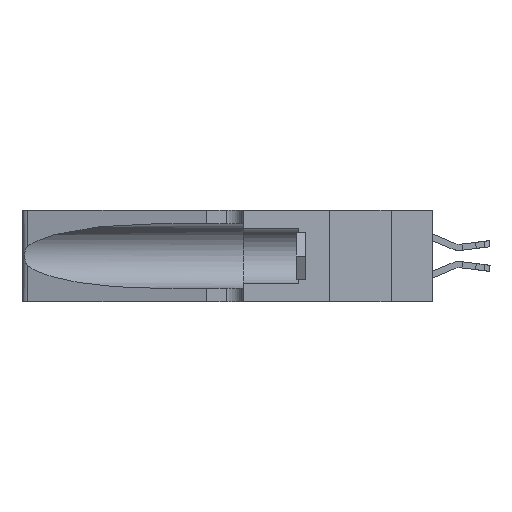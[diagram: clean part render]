
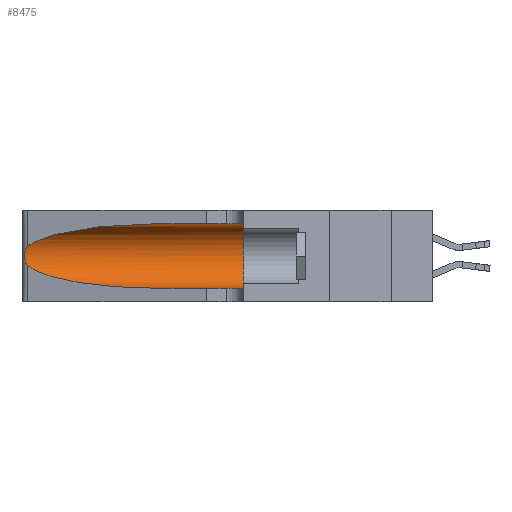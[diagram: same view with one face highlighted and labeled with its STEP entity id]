
A CAD part, left-side view. The second image highlights one B-rep face of the part: STEP entity #8475.
In plain terms, the highlighted cylindrical face has radius 3.308 mm (diameter 6.617 mm), a partial arc.
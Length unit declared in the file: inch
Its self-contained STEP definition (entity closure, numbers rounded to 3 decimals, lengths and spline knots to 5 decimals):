
#1839 = CARTESIAN_POINT ( 'NONE',  ( 0.1305, 0.35, 0.05475 ) ) ;
#1870 = CARTESIAN_POINT ( 'NONE',  ( 0.2373, 1.15595, 0.08982 ) ) ;
#2159 = CARTESIAN_POINT ( 'NONE',  ( 0.25856, 1.23593, 0.16098 ) ) ;
#3653 = LINE ( 'NONE', #21757, #31577 ) ;
#3708 = DIRECTION ( 'NONE',  ( 0., -1., 0. ) ) ;
#4135 = EDGE_CURVE ( 'NONE', #25041, #7422, #7489, .T. ) ;
#5105 = VECTOR ( 'NONE', #11735, 39.37008 ) ;
#5271 = CARTESIAN_POINT ( 'NONE',  ( 0.1305, 0.72297, 0.31525 ) ) ;
#5414 = VERTEX_POINT ( 'NONE', #26259 ) ;
#5548 = ORIENTED_EDGE ( 'NONE', *, *, #18888, .F. ) ;
#6478 = DIRECTION ( 'NONE',  ( 0., 1., 0. ) ) ;
#7023 = CARTESIAN_POINT ( 'NONE',  ( 0.25639, 1.23186, 0.15144 ) ) ;
#7106 = FACE_OUTER_BOUND ( 'NONE', #10210, .T. ) ;
#7422 = VERTEX_POINT ( 'NONE', #12897 ) ;
#7489 = B_SPLINE_CURVE_WITH_KNOTS ( 'NONE', 3,
 ( #26254, #9355, #31167, #16526, #26468, #31381, #23822, #11772, #9252, #2159, #31061, #7023, #16828, #28608 ),
 .UNSPECIFIED., .F., .F.,
 ( 4, 2, 2, 2, 2, 2, 4 ),
 ( 0., 0.00027, 0.00053, 0.00107, 0.0016, 0.00187, 0.00214 ),
 .UNSPECIFIED. ) ;
#8467 = DIRECTION ( 'NONE',  ( 0., 0., 1. ) ) ;
#8475 = ADVANCED_FACE ( 'NONE', ( #7106 ), #19738, .F. ) ;
#8517 = ORIENTED_EDGE ( 'NONE', *, *, #24353, .F. ) ;
#8689 = VERTEX_POINT ( 'NONE', #1839 ) ;
#9252 = CARTESIAN_POINT ( 'NONE',  ( 0.26017, 1.23833, 0.17102 ) ) ;
#9290 = ORIENTED_EDGE ( 'NONE', *, *, #15481, .T. ) ;
#9355 = CARTESIAN_POINT ( 'NONE',  ( 0.25555, 1.22994, 0.2215 ) ) ;
#9369 = EDGE_CURVE ( 'NONE', #5414, #8689, #11594, .T. ) ;
#10210 = EDGE_LOOP ( 'NONE', ( #9290, #16468, #14989, #31324, #5548, #8517 ) ) ;
#10294 = CARTESIAN_POINT ( 'NONE',  ( 0.25487, 1.22718, 0.22369 ) ) ;
#11476 = DIRECTION ( 'NONE',  ( 0., 0., -1. ) ) ;
#11594 = LINE ( 'NONE', #11845, #5105 ) ;
#11735 = DIRECTION ( 'NONE',  ( 0., -1., 0. ) ) ;
#11772 = CARTESIAN_POINT ( 'NONE',  ( 0.26075, 1.23896, 0.178 ) ) ;
#11845 = CARTESIAN_POINT ( 'NONE',  ( 0.1305, 1.61858, 0.05475 ) ) ;
#12417 = AXIS2_PLACEMENT_3D ( 'NONE', #27817, #3708, #11476 ) ;
#12897 = CARTESIAN_POINT ( 'NONE',  ( 0.25487, 1.22718, 0.14631 ) ) ;
#14813 = VERTEX_POINT ( 'NONE', #28020 ) ;
#14989 = ORIENTED_EDGE ( 'NONE', *, *, #23336, .T. ) ;
#15036 = AXIS2_PLACEMENT_3D ( 'NONE', #23365, #6478, #8467 ) ;
#15427 = CARTESIAN_POINT ( 'NONE',  ( 0.2373, 1.15595, 0.28018 ) ) ;
#15481 = EDGE_CURVE ( 'NONE', #31347, #25041, #19865, .T. ) ;
#16468 = ORIENTED_EDGE ( 'NONE', *, *, #4135, .T. ) ;
#16526 = CARTESIAN_POINT ( 'NONE',  ( 0.25787, 1.23484, 0.2124 ) ) ;
#16828 = CARTESIAN_POINT ( 'NONE',  ( 0.25555, 1.22993, 0.14849 ) ) ;
#17438 = CARTESIAN_POINT ( 'NONE',  ( 0.18966, 0.96281, 0.31525 ) ) ;
#18541 = CARTESIAN_POINT ( 'NONE',  ( 0.25487, 1.22718, 0.14631 ) ) ;
#18888 = EDGE_CURVE ( 'NONE', #14813, #8689, #31359, .T. ) ;
#18921 = CARTESIAN_POINT ( 'NONE',  ( 0.25487, 1.22718, 0.22369 ) ) ;
#19738 = CYLINDRICAL_SURFACE ( 'NONE', #12417, 0.13025 ) ;
#19865 =( BOUNDED_CURVE ( )  B_SPLINE_CURVE ( 3, ( #20535, #17438, #15427, #18921 ),
 .UNSPECIFIED., .F., .T. ) 
 B_SPLINE_CURVE_WITH_KNOTS ( ( 4, 4 ),
 ( 1.5708, 2.84003 ),
 .UNSPECIFIED. ) 
 CURVE ( )  GEOMETRIC_REPRESENTATION_ITEM ( )  RATIONAL_B_SPLINE_CURVE ( ( 1., 0.87, 0.87, 1. ) ) 
 REPRESENTATION_ITEM ( '' )  );
#20535 = CARTESIAN_POINT ( 'NONE',  ( 0.1305, 0.72297, 0.31525 ) ) ;
#21343 = DIRECTION ( 'NONE',  ( 0., -1., 0. ) ) ;
#21757 = CARTESIAN_POINT ( 'NONE',  ( 0.1305, 1.61858, 0.31525 ) ) ;
#23198 =( BOUNDED_CURVE ( )  B_SPLINE_CURVE ( 3, ( #18541, #1870, #27370, #27333 ),
 .UNSPECIFIED., .F., .F. ) 
 B_SPLINE_CURVE_WITH_KNOTS ( ( 4, 4 ),
 ( 3.44316, 4.71239 ),
 .UNSPECIFIED. ) 
 CURVE ( )  GEOMETRIC_REPRESENTATION_ITEM ( )  RATIONAL_B_SPLINE_CURVE ( ( 1., 0.87, 0.87, 1. ) ) 
 REPRESENTATION_ITEM ( '' )  );
#23336 = EDGE_CURVE ( 'NONE', #7422, #5414, #23198, .T. ) ;
#23365 = CARTESIAN_POINT ( 'NONE',  ( 0.1305, 0.35, 0.185 ) ) ;
#23822 = CARTESIAN_POINT ( 'NONE',  ( 0.26075, 1.23896, 0.19203 ) ) ;
#24353 = EDGE_CURVE ( 'NONE', #31347, #14813, #3653, .T. ) ;
#25041 = VERTEX_POINT ( 'NONE', #10294 ) ;
#26254 = CARTESIAN_POINT ( 'NONE',  ( 0.25487, 1.22718, 0.22369 ) ) ;
#26259 = CARTESIAN_POINT ( 'NONE',  ( 0.1305, 0.72297, 0.05475 ) ) ;
#26468 = CARTESIAN_POINT ( 'NONE',  ( 0.25854, 1.2359, 0.20912 ) ) ;
#27333 = CARTESIAN_POINT ( 'NONE',  ( 0.1305, 0.72297, 0.05475 ) ) ;
#27370 = CARTESIAN_POINT ( 'NONE',  ( 0.18966, 0.96281, 0.05475 ) ) ;
#27817 = CARTESIAN_POINT ( 'NONE',  ( 0.1305, 1.61858, 0.185 ) ) ;
#28020 = CARTESIAN_POINT ( 'NONE',  ( 0.1305, 0.35, 0.31525 ) ) ;
#28608 = CARTESIAN_POINT ( 'NONE',  ( 0.25487, 1.22718, 0.14631 ) ) ;
#31061 = CARTESIAN_POINT ( 'NONE',  ( 0.25789, 1.23486, 0.15765 ) ) ;
#31167 = CARTESIAN_POINT ( 'NONE',  ( 0.25639, 1.23184, 0.21858 ) ) ;
#31324 = ORIENTED_EDGE ( 'NONE', *, *, #9369, .T. ) ;
#31347 = VERTEX_POINT ( 'NONE', #5271 ) ;
#31359 = CIRCLE ( 'NONE', #15036, 0.13025 ) ;
#31381 = CARTESIAN_POINT ( 'NONE',  ( 0.26018, 1.23835, 0.19895 ) ) ;
#31577 = VECTOR ( 'NONE', #21343, 39.37008 ) ;
